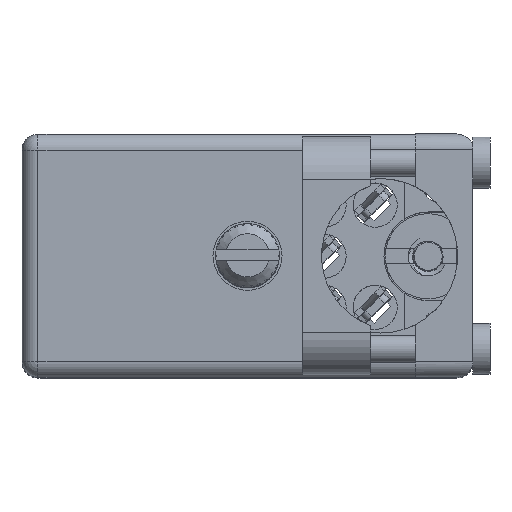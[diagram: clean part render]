
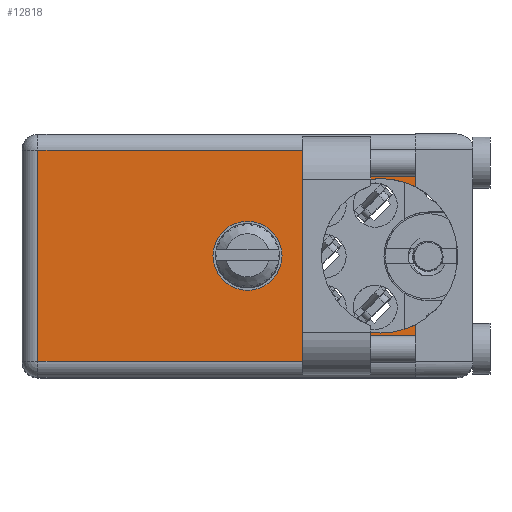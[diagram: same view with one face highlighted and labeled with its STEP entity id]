
A CAD part, top view. The second image highlights one B-rep face of the part: STEP entity #12818.
In plain terms, the highlighted face is planar.
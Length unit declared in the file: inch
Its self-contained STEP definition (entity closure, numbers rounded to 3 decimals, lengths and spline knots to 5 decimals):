
#2800 = VECTOR ( 'NONE', #179860, 39.37008 ) ;
#3608 = VERTEX_POINT ( 'NONE', #7791 ) ;
#6750 = CIRCLE ( 'NONE', #154122, 0.227 ) ;
#7539 = LINE ( 'NONE', #67398, #190683 ) ;
#7791 = CARTESIAN_POINT ( 'NONE',  ( 0.047, 0.906, -0.668 ) ) ;
#10910 = CARTESIAN_POINT ( 'NONE',  ( 1.155, 0.906, 0. ) ) ;
#11583 = FACE_OUTER_BOUND ( 'NONE', #15386, .T. ) ;
#12182 = EDGE_CURVE ( 'NONE', #180677, #76968, #53577, .T. ) ;
#12578 = DIRECTION ( 'NONE',  ( 0., 1., 0. ) ) ;
#12818 = ADVANCED_FACE ( 'NONE', ( #11583, #131425 ), #116702, .T. ) ;
#13164 = DIRECTION ( 'NONE',  ( 0., 1., 0. ) ) ;
#15386 = EDGE_LOOP ( 'NONE', ( #80205, #51261, #111499, #88444, #84455, #77841, #123177, #47506 ) ) ;
#19157 = AXIS2_PLACEMENT_3D ( 'NONE', #29256, #12578, #176622 ) ;
#20972 = CARTESIAN_POINT ( 'NONE',  ( 1.155, 0.906, -0.047 ) ) ;
#22574 = EDGE_CURVE ( 'NONE', #113142, #188218, #117247, .T. ) ;
#23598 = CARTESIAN_POINT ( 'NONE',  ( 1.053, 0.906, -0.3575 ) ) ;
#24126 = DIRECTION ( 'NONE',  ( 0., 0., 1. ) ) ;
#26627 = DIRECTION ( 'NONE',  ( 0., 0., 1. ) ) ;
#29181 = EDGE_CURVE ( 'NONE', #129249, #102629, #7539, .T. ) ;
#29256 = CARTESIAN_POINT ( 'NONE',  ( 0., 0.906, -0.715 ) ) ;
#41254 = DIRECTION ( 'NONE',  ( 0., 0., 1. ) ) ;
#41322 = CARTESIAN_POINT ( 'NONE',  ( 0.6625, 0.906, -0.3575 ) ) ;
#42289 = DIRECTION ( 'NONE',  ( 0., 0., 1. ) ) ;
#47506 = ORIENTED_EDGE ( 'NONE', *, *, #60956, .F. ) ;
#51261 = ORIENTED_EDGE ( 'NONE', *, *, #62257, .T. ) ;
#52011 = AXIS2_PLACEMENT_3D ( 'NONE', #41322, #105157, #42289 ) ;
#53577 = CIRCLE ( 'NONE', #100593, 0.1015 ) ;
#55848 = VECTOR ( 'NONE', #26627, 39.37008 ) ;
#56661 = CARTESIAN_POINT ( 'NONE',  ( 1.053, 0.906, -0.5845 ) ) ;
#60585 = LINE ( 'NONE', #118625, #182322 ) ;
#60956 = EDGE_CURVE ( 'NONE', #186242, #113142, #6750, .T. ) ;
#62257 = EDGE_CURVE ( 'NONE', #96737, #3608, #60585, .T. ) ;
#65626 = DIRECTION ( 'NONE',  ( 0., 0., 1. ) ) ;
#67398 = CARTESIAN_POINT ( 'NONE',  ( 1.155, 0.906, -0.047 ) ) ;
#67601 = EDGE_CURVE ( 'NONE', #3608, #129249, #86420, .T. ) ;
#70679 = DIRECTION ( 'NONE',  ( 0., 1., 0. ) ) ;
#71259 = ORIENTED_EDGE ( 'NONE', *, *, #12182, .F. ) ;
#75357 = DIRECTION ( 'NONE',  ( -1., 0., 0. ) ) ;
#76968 = VERTEX_POINT ( 'NONE', #136164 ) ;
#77841 = ORIENTED_EDGE ( 'NONE', *, *, #88421, .F. ) ;
#79481 = AXIS2_PLACEMENT_3D ( 'NONE', #147733, #13164, #150626 ) ;
#80205 = ORIENTED_EDGE ( 'NONE', *, *, #192066, .F. ) ;
#80991 = VERTEX_POINT ( 'NONE', #109725 ) ;
#82072 = CARTESIAN_POINT ( 'NONE',  ( 1.053, 0.906, -0.3575 ) ) ;
#84005 = DIRECTION ( 'NONE',  ( 0., 1., 0. ) ) ;
#84455 = ORIENTED_EDGE ( 'NONE', *, *, #153200, .F. ) ;
#86420 = LINE ( 'NONE', #89337, #90996 ) ;
#88421 = EDGE_CURVE ( 'NONE', #188218, #80991, #165149, .T. ) ;
#88444 = ORIENTED_EDGE ( 'NONE', *, *, #29181, .T. ) ;
#89337 = CARTESIAN_POINT ( 'NONE',  ( 0.047, 0.906, -0.715 ) ) ;
#89443 = LINE ( 'NONE', #176948, #2800 ) ;
#90996 = VECTOR ( 'NONE', #41254, 39.37008 ) ;
#96737 = VERTEX_POINT ( 'NONE', #128052 ) ;
#100593 = AXIS2_PLACEMENT_3D ( 'NONE', #141318, #132144, #65626 ) ;
#102629 = VERTEX_POINT ( 'NONE', #20972 ) ;
#105157 = DIRECTION ( 'NONE',  ( 0., 1., 0. ) ) ;
#105383 = CIRCLE ( 'NONE', #52011, 0.1015 ) ;
#108278 = EDGE_LOOP ( 'NONE', ( #185148, #71259 ) ) ;
#109725 = CARTESIAN_POINT ( 'NONE',  ( 1.155, 0.906, -0.15471 ) ) ;
#111499 = ORIENTED_EDGE ( 'NONE', *, *, #67601, .T. ) ;
#112138 = LINE ( 'NONE', #10910, #55848 ) ;
#112247 = CARTESIAN_POINT ( 'NONE',  ( 1.053, 0.906, -0.1305 ) ) ;
#113142 = VERTEX_POINT ( 'NONE', #56661 ) ;
#113845 = CARTESIAN_POINT ( 'NONE',  ( 0.047, 0.906, -0.047 ) ) ;
#114907 = AXIS2_PLACEMENT_3D ( 'NONE', #23598, #70679, #129645 ) ;
#116702 = PLANE ( 'NONE',  #19157 ) ;
#117247 = CIRCLE ( 'NONE', #79481, 0.227 ) ;
#118625 = CARTESIAN_POINT ( 'NONE',  ( 0., 0.906, -0.668 ) ) ;
#118760 = CARTESIAN_POINT ( 'NONE',  ( 0.6625, 0.906, -0.459 ) ) ;
#119647 = CARTESIAN_POINT ( 'NONE',  ( 1.155, 0.906, -0.56029 ) ) ;
#121568 = EDGE_CURVE ( 'NONE', #76968, #180677, #105383, .T. ) ;
#123177 = ORIENTED_EDGE ( 'NONE', *, *, #22574, .F. ) ;
#128052 = CARTESIAN_POINT ( 'NONE',  ( 1.155, 0.906, -0.668 ) ) ;
#129249 = VERTEX_POINT ( 'NONE', #113845 ) ;
#129645 = DIRECTION ( 'NONE',  ( 0., 0., 1. ) ) ;
#131425 = FACE_BOUND ( 'NONE', #108278, .T. ) ;
#132144 = DIRECTION ( 'NONE',  ( 0., 1., 0. ) ) ;
#136164 = CARTESIAN_POINT ( 'NONE',  ( 0.6625, 0.906, -0.256 ) ) ;
#141318 = CARTESIAN_POINT ( 'NONE',  ( 0.6625, 0.906, -0.3575 ) ) ;
#147733 = CARTESIAN_POINT ( 'NONE',  ( 1.053, 0.906, -0.3575 ) ) ;
#150626 = DIRECTION ( 'NONE',  ( 0., 0., 1. ) ) ;
#153200 = EDGE_CURVE ( 'NONE', #80991, #102629, #89443, .T. ) ;
#154122 = AXIS2_PLACEMENT_3D ( 'NONE', #82072, #84005, #24126 ) ;
#157806 = DIRECTION ( 'NONE',  ( 1., 0., 0. ) ) ;
#165149 = CIRCLE ( 'NONE', #114907, 0.227 ) ;
#176622 = DIRECTION ( 'NONE',  ( 0., 0., 1. ) ) ;
#176948 = CARTESIAN_POINT ( 'NONE',  ( 1.155, 0.906, 0. ) ) ;
#179860 = DIRECTION ( 'NONE',  ( 0., 0., 1. ) ) ;
#180677 = VERTEX_POINT ( 'NONE', #118760 ) ;
#182322 = VECTOR ( 'NONE', #75357, 39.37008 ) ;
#185148 = ORIENTED_EDGE ( 'NONE', *, *, #121568, .F. ) ;
#186242 = VERTEX_POINT ( 'NONE', #119647 ) ;
#188218 = VERTEX_POINT ( 'NONE', #112247 ) ;
#190683 = VECTOR ( 'NONE', #157806, 39.37008 ) ;
#192066 = EDGE_CURVE ( 'NONE', #96737, #186242, #112138, .T. ) ;
